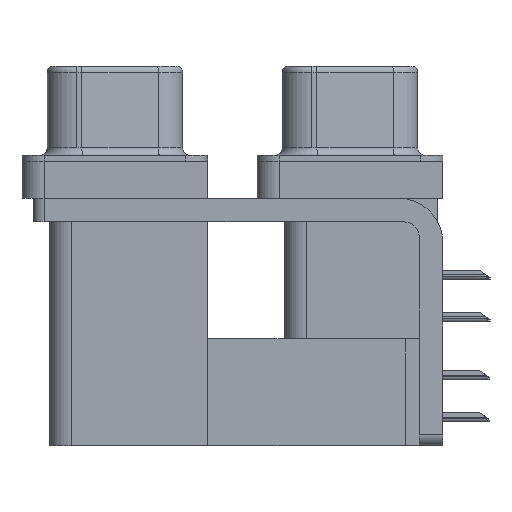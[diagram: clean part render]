
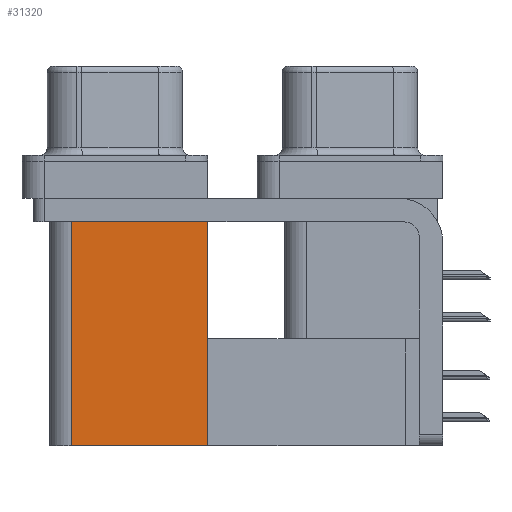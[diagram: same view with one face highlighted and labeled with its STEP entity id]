
A CAD part, left-side view. The second image highlights one B-rep face of the part: STEP entity #31320.
In plain terms, the highlighted planar face has unit normal (-1, 0, 0).
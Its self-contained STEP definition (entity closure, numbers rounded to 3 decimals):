
#227 = LINE ( 'NONE', #41341, #21138 ) ;
#836 = DIRECTION ( 'NONE',  ( 0., 0., -1. ) ) ;
#1489 = EDGE_LOOP ( 'NONE', ( #12374, #13752, #12426, #38998 ) ) ;
#5616 = VERTEX_POINT ( 'NONE', #28800 ) ;
#6097 = LINE ( 'NONE', #17850, #16568 ) ;
#8064 = CARTESIAN_POINT ( 'NONE',  ( 3.79, 18.8, -19.2 ) ) ;
#11848 = FACE_OUTER_BOUND ( 'NONE', #1489, .T. ) ;
#12374 = ORIENTED_EDGE ( 'NONE', *, *, #37987, .T. ) ;
#12426 = ORIENTED_EDGE ( 'NONE', *, *, #19119, .F. ) ;
#13752 = ORIENTED_EDGE ( 'NONE', *, *, #32189, .F. ) ;
#16011 = CARTESIAN_POINT ( 'NONE',  ( 3.79, 9.6, -19.2 ) ) ;
#16568 = VECTOR ( 'NONE', #21301, 1000. ) ;
#17850 = CARTESIAN_POINT ( 'NONE',  ( 3.79, 9.6, -19.2 ) ) ;
#17998 = VERTEX_POINT ( 'NONE', #30203 ) ;
#18613 = DIRECTION ( 'NONE',  ( 0., 0., 1. ) ) ;
#19119 = EDGE_CURVE ( 'NONE', #17998, #46997, #227, .T. ) ;
#21138 = VECTOR ( 'NONE', #34501, 1000. ) ;
#21301 = DIRECTION ( 'NONE',  ( 0., 0., 1. ) ) ;
#28450 = LINE ( 'NONE', #32608, #33741 ) ;
#28667 = AXIS2_PLACEMENT_3D ( 'NONE', #16011, #38304, #836 ) ;
#28800 = CARTESIAN_POINT ( 'NONE',  ( 3.79, 18.8, -2.5 ) ) ;
#30102 = LINE ( 'NONE', #8064, #33424 ) ;
#30203 = CARTESIAN_POINT ( 'NONE',  ( 3.79, 9.6, -19.2 ) ) ;
#31320 = ADVANCED_FACE ( 'NONE', ( #11848 ), #41230, .F. ) ;
#32189 = EDGE_CURVE ( 'NONE', #46997, #5616, #30102, .T. ) ;
#32608 = CARTESIAN_POINT ( 'NONE',  ( 3.79, 9.6, -2.5 ) ) ;
#33424 = VECTOR ( 'NONE', #18613, 1000. ) ;
#33741 = VECTOR ( 'NONE', #47526, 1000. ) ;
#34330 = CARTESIAN_POINT ( 'NONE',  ( 3.79, 18.8, -19.2 ) ) ;
#34501 = DIRECTION ( 'NONE',  ( 0., 1., 0. ) ) ;
#37987 = EDGE_CURVE ( 'NONE', #43928, #5616, #28450, .T. ) ;
#38304 = DIRECTION ( 'NONE',  ( 1., 0., 0. ) ) ;
#38519 = EDGE_CURVE ( 'NONE', #17998, #43928, #6097, .T. ) ;
#38998 = ORIENTED_EDGE ( 'NONE', *, *, #38519, .T. ) ;
#41230 = PLANE ( 'NONE',  #28667 ) ;
#41341 = CARTESIAN_POINT ( 'NONE',  ( 3.79, 9.6, -19.2 ) ) ;
#43928 = VERTEX_POINT ( 'NONE', #46181 ) ;
#46181 = CARTESIAN_POINT ( 'NONE',  ( 3.79, 9.6, -2.5 ) ) ;
#46997 = VERTEX_POINT ( 'NONE', #34330 ) ;
#47526 = DIRECTION ( 'NONE',  ( 0., 1., 0. ) ) ;
